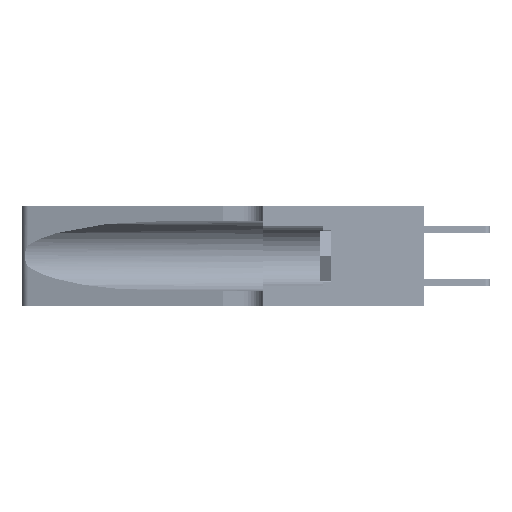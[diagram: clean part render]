
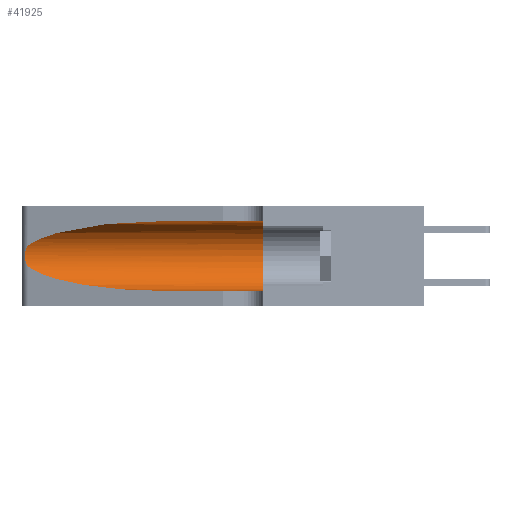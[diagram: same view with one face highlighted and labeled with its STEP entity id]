
A CAD part, left-side view. The second image highlights one B-rep face of the part: STEP entity #41925.
In plain terms, the highlighted cylindrical face has radius 3.308 mm (diameter 6.617 mm), a partial arc.
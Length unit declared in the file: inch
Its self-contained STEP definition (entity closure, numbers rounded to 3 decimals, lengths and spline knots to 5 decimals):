
#647 = CIRCLE ( 'NONE', #5829, 0.13025 ) ;
#1116 = AXIS2_PLACEMENT_3D ( 'NONE', #3462, #40300, #20416 ) ;
#1165 = CARTESIAN_POINT ( 'NONE',  ( 0.18966, 0.96281, 0.05475 ) ) ;
#1488 = CARTESIAN_POINT ( 'NONE',  ( 0.2373, 1.15595, 0.08982 ) ) ;
#1721 = DIRECTION ( 'NONE',  ( 0., 1., 0. ) ) ;
#2536 = CARTESIAN_POINT ( 'NONE',  ( 0.25639, 1.23186, 0.15144 ) ) ;
#3462 = CARTESIAN_POINT ( 'NONE',  ( 0.1305, 1.61858, 0.185 ) ) ;
#3625 = CYLINDRICAL_SURFACE ( 'NONE', #1116, 0.13025 ) ;
#3735 = LINE ( 'NONE', #20085, #36961 ) ;
#4010 = LINE ( 'NONE', #8468, #35752 ) ;
#4128 = FACE_OUTER_BOUND ( 'NONE', #15927, .T. ) ;
#4921 = CARTESIAN_POINT ( 'NONE',  ( 0.1305, 0.35, 0.31525 ) ) ;
#5183 = DIRECTION ( 'NONE',  ( 0., 0., 1. ) ) ;
#5829 = AXIS2_PLACEMENT_3D ( 'NONE', #28510, #1721, #5183 ) ;
#6591 = ORIENTED_EDGE ( 'NONE', *, *, #7401, .T. ) ;
#7401 = EDGE_CURVE ( 'NONE', #24352, #15643, #11275, .T. ) ;
#8468 = CARTESIAN_POINT ( 'NONE',  ( 0.1305, 1.61858, 0.05475 ) ) ;
#8654 = ORIENTED_EDGE ( 'NONE', *, *, #34388, .T. ) ;
#9187 = CARTESIAN_POINT ( 'NONE',  ( 0.25487, 1.22718, 0.14631 ) ) ;
#9969 = CARTESIAN_POINT ( 'NONE',  ( 0.1305, 0.72297, 0.31525 ) ) ;
#10007 = ORIENTED_EDGE ( 'NONE', *, *, #20410, .T. ) ;
#11275 =( BOUNDED_CURVE ( )  B_SPLINE_CURVE ( 3, ( #37535, #1488, #1165, #11441 ),
 .UNSPECIFIED., .F., .F. ) 
 B_SPLINE_CURVE_WITH_KNOTS ( ( 4, 4 ),
 ( 3.44316, 4.71239 ),
 .UNSPECIFIED. ) 
 CURVE ( )  GEOMETRIC_REPRESENTATION_ITEM ( )  RATIONAL_B_SPLINE_CURVE ( ( 1., 0.87, 0.87, 1. ) ) 
 REPRESENTATION_ITEM ( '' )  );
#11441 = CARTESIAN_POINT ( 'NONE',  ( 0.1305, 0.72297, 0.05475 ) ) ;
#11820 = ORIENTED_EDGE ( 'NONE', *, *, #40492, .F. ) ;
#12373 = CARTESIAN_POINT ( 'NONE',  ( 0.25854, 1.2359, 0.20912 ) ) ;
#12892 = EDGE_CURVE ( 'NONE', #40419, #37974, #3735, .T. ) ;
#14705 = CARTESIAN_POINT ( 'NONE',  ( 0.1305, 0.35, 0.05475 ) ) ;
#15643 = VERTEX_POINT ( 'NONE', #21293 ) ;
#15927 = EDGE_LOOP ( 'NONE', ( #10007, #38634, #6591, #8654, #11820, #35186 ) ) ;
#18782 = CARTESIAN_POINT ( 'NONE',  ( 0.26075, 1.23896, 0.178 ) ) ;
#18923 = CARTESIAN_POINT ( 'NONE',  ( 0.25639, 1.23184, 0.21858 ) ) ;
#19057 = CARTESIAN_POINT ( 'NONE',  ( 0.25789, 1.23486, 0.15765 ) ) ;
#19420 = CARTESIAN_POINT ( 'NONE',  ( 0.2373, 1.15595, 0.28018 ) ) ;
#19527 =( BOUNDED_CURVE ( )  B_SPLINE_CURVE ( 3, ( #9969, #33203, #19420, #42766 ),
 .UNSPECIFIED., .F., .T. ) 
 B_SPLINE_CURVE_WITH_KNOTS ( ( 4, 4 ),
 ( 1.5708, 2.84003 ),
 .UNSPECIFIED. ) 
 CURVE ( )  GEOMETRIC_REPRESENTATION_ITEM ( )  RATIONAL_B_SPLINE_CURVE ( ( 1., 0.87, 0.87, 1. ) ) 
 REPRESENTATION_ITEM ( '' )  );
#20085 = CARTESIAN_POINT ( 'NONE',  ( 0.1305, 1.61858, 0.31525 ) ) ;
#20410 = EDGE_CURVE ( 'NONE', #40419, #25421, #19527, .T. ) ;
#20416 = DIRECTION ( 'NONE',  ( 0., 0., -1. ) ) ;
#21293 = CARTESIAN_POINT ( 'NONE',  ( 0.1305, 0.72297, 0.05475 ) ) ;
#21985 = CARTESIAN_POINT ( 'NONE',  ( 0.25555, 1.22994, 0.2215 ) ) ;
#22400 = CARTESIAN_POINT ( 'NONE',  ( 0.25487, 1.22718, 0.22369 ) ) ;
#22423 = DIRECTION ( 'NONE',  ( 0., -1., 0. ) ) ;
#24352 = VERTEX_POINT ( 'NONE', #28104 ) ;
#24484 = CARTESIAN_POINT ( 'NONE',  ( 0.25487, 1.22718, 0.22369 ) ) ;
#25319 = CARTESIAN_POINT ( 'NONE',  ( 0.25555, 1.22993, 0.14849 ) ) ;
#25418 = B_SPLINE_CURVE_WITH_KNOTS ( 'NONE', 3,
 ( #22400, #21985, #18923, #35337, #12373, #38957, #38671, #18782, #28793, #35621, #19057, #2536, #25319, #9187 ),
 .UNSPECIFIED., .F., .F.,
 ( 4, 2, 2, 2, 2, 2, 4 ),
 ( 0., 0.00027, 0.00053, 0.00107, 0.0016, 0.00187, 0.00214 ),
 .UNSPECIFIED. ) ;
#25421 = VERTEX_POINT ( 'NONE', #24484 ) ;
#26947 = EDGE_CURVE ( 'NONE', #25421, #24352, #25418, .T. ) ;
#28104 = CARTESIAN_POINT ( 'NONE',  ( 0.25487, 1.22718, 0.14631 ) ) ;
#28489 = DIRECTION ( 'NONE',  ( 0., -1., 0. ) ) ;
#28510 = CARTESIAN_POINT ( 'NONE',  ( 0.1305, 0.35, 0.185 ) ) ;
#28793 = CARTESIAN_POINT ( 'NONE',  ( 0.26017, 1.23833, 0.17102 ) ) ;
#33203 = CARTESIAN_POINT ( 'NONE',  ( 0.18966, 0.96281, 0.31525 ) ) ;
#34388 = EDGE_CURVE ( 'NONE', #15643, #37619, #4010, .T. ) ;
#34749 = CARTESIAN_POINT ( 'NONE',  ( 0.1305, 0.72297, 0.31525 ) ) ;
#35186 = ORIENTED_EDGE ( 'NONE', *, *, #12892, .F. ) ;
#35337 = CARTESIAN_POINT ( 'NONE',  ( 0.25787, 1.23484, 0.2124 ) ) ;
#35621 = CARTESIAN_POINT ( 'NONE',  ( 0.25856, 1.23593, 0.16098 ) ) ;
#35752 = VECTOR ( 'NONE', #28489, 39.37008 ) ;
#36961 = VECTOR ( 'NONE', #22423, 39.37008 ) ;
#37535 = CARTESIAN_POINT ( 'NONE',  ( 0.25487, 1.22718, 0.14631 ) ) ;
#37619 = VERTEX_POINT ( 'NONE', #14705 ) ;
#37974 = VERTEX_POINT ( 'NONE', #4921 ) ;
#38634 = ORIENTED_EDGE ( 'NONE', *, *, #26947, .T. ) ;
#38671 = CARTESIAN_POINT ( 'NONE',  ( 0.26075, 1.23896, 0.19203 ) ) ;
#38957 = CARTESIAN_POINT ( 'NONE',  ( 0.26018, 1.23835, 0.19895 ) ) ;
#40300 = DIRECTION ( 'NONE',  ( 0., -1., 0. ) ) ;
#40419 = VERTEX_POINT ( 'NONE', #34749 ) ;
#40492 = EDGE_CURVE ( 'NONE', #37974, #37619, #647, .T. ) ;
#41925 = ADVANCED_FACE ( 'NONE', ( #4128 ), #3625, .F. ) ;
#42766 = CARTESIAN_POINT ( 'NONE',  ( 0.25487, 1.22718, 0.22369 ) ) ;
